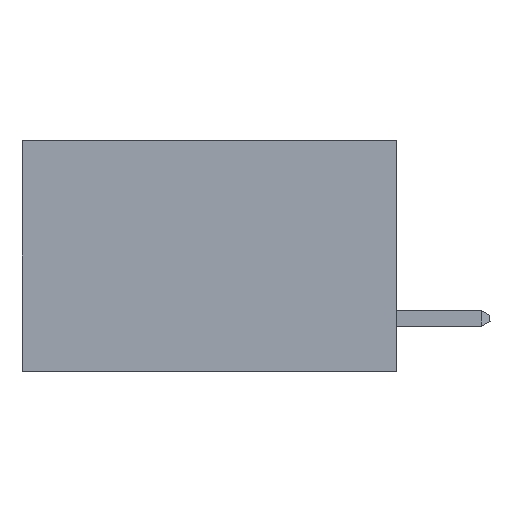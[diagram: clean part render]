
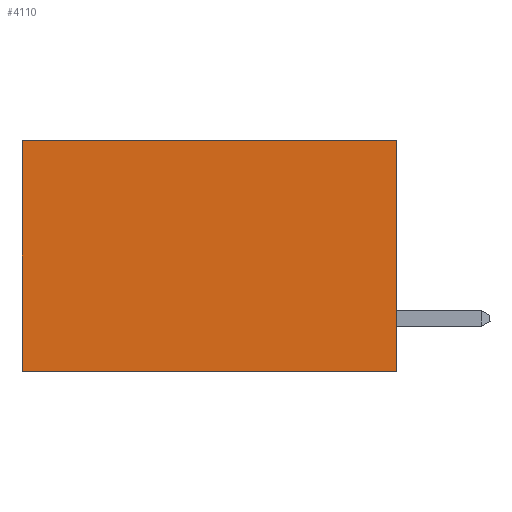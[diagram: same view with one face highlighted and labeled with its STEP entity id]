
A CAD part, left-side view. The second image highlights one B-rep face of the part: STEP entity #4110.
In plain terms, the highlighted planar face has unit normal (-1, 0, 0).
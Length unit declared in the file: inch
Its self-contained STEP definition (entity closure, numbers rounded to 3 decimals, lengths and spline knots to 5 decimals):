
#918 = DIRECTION ( 'NONE',  ( 0., 0., -1. ) ) ;
#1600 = LINE ( 'NONE', #8292, #7670 ) ;
#1605 = ORIENTED_EDGE ( 'NONE', *, *, #9764, .T. ) ;
#1683 = DIRECTION ( 'NONE',  ( 0., 1., 0. ) ) ;
#2370 = VERTEX_POINT ( 'NONE', #12919 ) ;
#2739 = CARTESIAN_POINT ( 'NONE',  ( 0.298, 0., -0.37 ) ) ;
#3041 = FACE_OUTER_BOUND ( 'NONE', #25069, .T. ) ;
#4110 = ADVANCED_FACE ( 'NONE', ( #3041 ), #12793, .F. ) ;
#5499 = LINE ( 'NONE', #7257, #22975 ) ;
#6371 = CARTESIAN_POINT ( 'NONE',  ( 0.298, 0.6, 0. ) ) ;
#7257 = CARTESIAN_POINT ( 'NONE',  ( 0.298, 0., 0. ) ) ;
#7455 = ORIENTED_EDGE ( 'NONE', *, *, #10274, .T. ) ;
#7670 = VECTOR ( 'NONE', #1683, 39.37008 ) ;
#8292 = CARTESIAN_POINT ( 'NONE',  ( 0.298, 0., -0.37 ) ) ;
#8840 = CARTESIAN_POINT ( 'NONE',  ( 0.298, 0.6, 0. ) ) ;
#9764 = EDGE_CURVE ( 'NONE', #2370, #11750, #27331, .T. ) ;
#10274 = EDGE_CURVE ( 'NONE', #11750, #17148, #19572, .T. ) ;
#10549 = DIRECTION ( 'NONE',  ( 0., 0., -1. ) ) ;
#11537 = AXIS2_PLACEMENT_3D ( 'NONE', #23393, #23302, #10549 ) ;
#11750 = VERTEX_POINT ( 'NONE', #8840 ) ;
#12793 = PLANE ( 'NONE',  #11537 ) ;
#12833 = ORIENTED_EDGE ( 'NONE', *, *, #17989, .F. ) ;
#12919 = CARTESIAN_POINT ( 'NONE',  ( 0.298, 0., 0. ) ) ;
#13030 = DIRECTION ( 'NONE',  ( 0., 1., 0. ) ) ;
#13571 = VERTEX_POINT ( 'NONE', #2739 ) ;
#15337 = EDGE_CURVE ( 'NONE', #2370, #13571, #5499, .T. ) ;
#15905 = VECTOR ( 'NONE', #13030, 39.37008 ) ;
#17148 = VERTEX_POINT ( 'NONE', #19476 ) ;
#17989 = EDGE_CURVE ( 'NONE', #13571, #17148, #1600, .T. ) ;
#19476 = CARTESIAN_POINT ( 'NONE',  ( 0.298, 0.6, -0.37 ) ) ;
#19572 = LINE ( 'NONE', #6371, #21246 ) ;
#19886 = ORIENTED_EDGE ( 'NONE', *, *, #15337, .F. ) ;
#21246 = VECTOR ( 'NONE', #27898, 39.37008 ) ;
#21284 = CARTESIAN_POINT ( 'NONE',  ( 0.298, 0., 0. ) ) ;
#22975 = VECTOR ( 'NONE', #918, 39.37008 ) ;
#23302 = DIRECTION ( 'NONE',  ( 1., 0., 0. ) ) ;
#23393 = CARTESIAN_POINT ( 'NONE',  ( 0.298, 0., 0. ) ) ;
#25069 = EDGE_LOOP ( 'NONE', ( #7455, #12833, #19886, #1605 ) ) ;
#27331 = LINE ( 'NONE', #21284, #15905 ) ;
#27898 = DIRECTION ( 'NONE',  ( 0., 0., -1. ) ) ;
